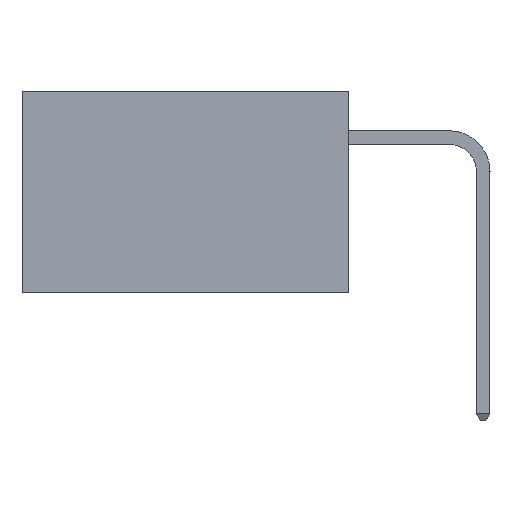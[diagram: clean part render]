
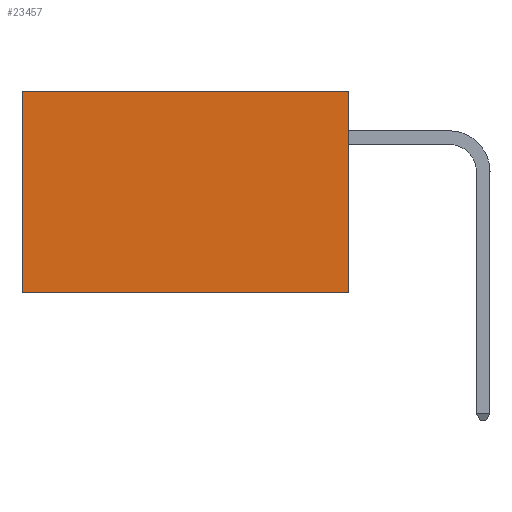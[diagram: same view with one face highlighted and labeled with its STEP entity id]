
A CAD part, left-side view. The second image highlights one B-rep face of the part: STEP entity #23457.
In plain terms, the highlighted planar face has unit normal (-1, 0, 0).
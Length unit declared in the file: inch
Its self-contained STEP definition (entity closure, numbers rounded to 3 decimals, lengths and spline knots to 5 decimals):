
#1237 = DIRECTION ( 'NONE',  ( 0., 0., -1. ) ) ;
#2798 = EDGE_CURVE ( 'NONE', #3421, #6963, #22451, .T. ) ;
#3421 = VERTEX_POINT ( 'NONE', #10135 ) ;
#3659 = ORIENTED_EDGE ( 'NONE', *, *, #21653, .T. ) ;
#4840 = LINE ( 'NONE', #13419, #14729 ) ;
#5701 = DIRECTION ( 'NONE',  ( 0., 0., -1. ) ) ;
#6765 = DIRECTION ( 'NONE',  ( 0., 1., 0. ) ) ;
#6963 = VERTEX_POINT ( 'NONE', #7541 ) ;
#7034 = VECTOR ( 'NONE', #6765, 39.37008 ) ;
#7259 = CARTESIAN_POINT ( 'NONE',  ( 0.2875, 0.6, 0. ) ) ;
#7541 = CARTESIAN_POINT ( 'NONE',  ( 0.2875, 0.6, 0. ) ) ;
#7598 = VERTEX_POINT ( 'NONE', #13908 ) ;
#9220 = VERTEX_POINT ( 'NONE', #9843 ) ;
#9242 = EDGE_CURVE ( 'NONE', #7598, #9220, #14867, .T. ) ;
#9493 = FACE_OUTER_BOUND ( 'NONE', #20530, .T. ) ;
#9808 = AXIS2_PLACEMENT_3D ( 'NONE', #23038, #17408, #5701 ) ;
#9843 = CARTESIAN_POINT ( 'NONE',  ( 0.2875, 0.6, -0.37 ) ) ;
#9966 = ORIENTED_EDGE ( 'NONE', *, *, #2798, .T. ) ;
#10135 = CARTESIAN_POINT ( 'NONE',  ( 0.2875, 0., 0. ) ) ;
#11784 = ORIENTED_EDGE ( 'NONE', *, *, #23397, .F. ) ;
#13419 = CARTESIAN_POINT ( 'NONE',  ( 0.2875, 0., 0. ) ) ;
#13583 = PLANE ( 'NONE',  #9808 ) ;
#13908 = CARTESIAN_POINT ( 'NONE',  ( 0.2875, 0., -0.37 ) ) ;
#14254 = VECTOR ( 'NONE', #15832, 39.37008 ) ;
#14729 = VECTOR ( 'NONE', #15355, 39.37008 ) ;
#14867 = LINE ( 'NONE', #21455, #14254 ) ;
#15355 = DIRECTION ( 'NONE',  ( 0., 0., -1. ) ) ;
#15832 = DIRECTION ( 'NONE',  ( 0., 1., 0. ) ) ;
#16015 = VECTOR ( 'NONE', #1237, 39.37008 ) ;
#16610 = LINE ( 'NONE', #7259, #16015 ) ;
#17408 = DIRECTION ( 'NONE',  ( 1., 0., 0. ) ) ;
#18449 = CARTESIAN_POINT ( 'NONE',  ( 0.2875, 0., 0. ) ) ;
#20348 = ORIENTED_EDGE ( 'NONE', *, *, #9242, .F. ) ;
#20530 = EDGE_LOOP ( 'NONE', ( #3659, #20348, #11784, #9966 ) ) ;
#21455 = CARTESIAN_POINT ( 'NONE',  ( 0.2875, 0., -0.37 ) ) ;
#21653 = EDGE_CURVE ( 'NONE', #6963, #9220, #16610, .T. ) ;
#22451 = LINE ( 'NONE', #18449, #7034 ) ;
#23038 = CARTESIAN_POINT ( 'NONE',  ( 0.2875, 0., 0. ) ) ;
#23397 = EDGE_CURVE ( 'NONE', #3421, #7598, #4840, .T. ) ;
#23457 = ADVANCED_FACE ( 'NONE', ( #9493 ), #13583, .F. ) ;
